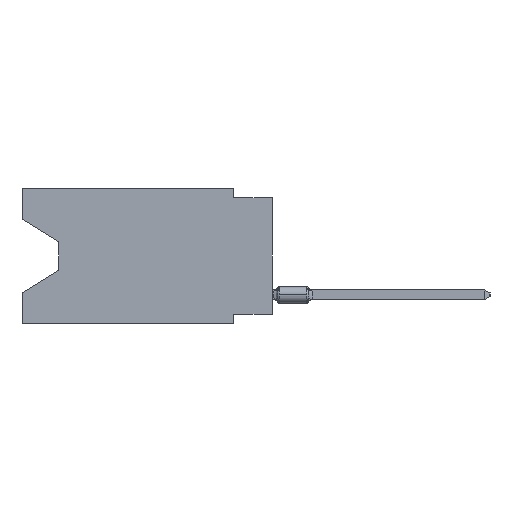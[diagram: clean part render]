
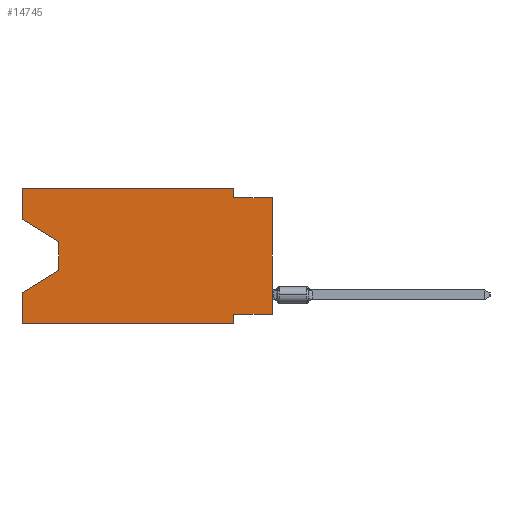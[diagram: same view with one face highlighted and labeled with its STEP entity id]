
A CAD part, left-side view. The second image highlights one B-rep face of the part: STEP entity #14745.
In plain terms, the highlighted planar face has unit normal (-1, 0, 0).
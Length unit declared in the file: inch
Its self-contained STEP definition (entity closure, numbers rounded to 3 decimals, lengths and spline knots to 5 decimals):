
#199 = ORIENTED_EDGE ( 'NONE', *, *, #22991, .T. ) ;
#1164 = CARTESIAN_POINT ( 'NONE',  ( 0., 0., -0.025 ) ) ;
#1546 = VERTEX_POINT ( 'NONE', #31990 ) ;
#1868 = CARTESIAN_POINT ( 'NONE',  ( 0., 0.645, 0. ) ) ;
#2002 = LINE ( 'NONE', #14101, #34055 ) ;
#2009 = VECTOR ( 'NONE', #32151, 39.37008 ) ;
#3242 = EDGE_CURVE ( 'NONE', #35832, #35520, #16876, .T. ) ;
#3734 = EDGE_CURVE ( 'NONE', #18222, #15809, #5132, .T. ) ;
#4199 = VERTEX_POINT ( 'NONE', #38492 ) ;
#4399 = CARTESIAN_POINT ( 'NONE',  ( 0., 0.1, -0.325 ) ) ;
#4623 = CARTESIAN_POINT ( 'NONE',  ( 0., 0., -0.325 ) ) ;
#4688 = EDGE_CURVE ( 'NONE', #5447, #1546, #36260, .T. ) ;
#5040 = CARTESIAN_POINT ( 'NONE',  ( 0., 0.645, -0.08025 ) ) ;
#5132 = LINE ( 'NONE', #23923, #17165 ) ;
#5334 = ORIENTED_EDGE ( 'NONE', *, *, #19555, .T. ) ;
#5447 = VERTEX_POINT ( 'NONE', #22988 ) ;
#5611 = DIRECTION ( 'NONE',  ( 0., -1., 0. ) ) ;
#5726 = VERTEX_POINT ( 'NONE', #40575 ) ;
#6654 = LINE ( 'NONE', #32352, #2009 ) ;
#6931 = LINE ( 'NONE', #4623, #17175 ) ;
#7635 = DIRECTION ( 'NONE',  ( 0., -1., 0. ) ) ;
#8269 = DIRECTION ( 'NONE',  ( 0., 0., -1. ) ) ;
#8431 = DIRECTION ( 'NONE',  ( 0., 0., -1. ) ) ;
#8499 = VERTEX_POINT ( 'NONE', #1868 ) ;
#9174 = ORIENTED_EDGE ( 'NONE', *, *, #12309, .T. ) ;
#11509 = ORIENTED_EDGE ( 'NONE', *, *, #4688, .F. ) ;
#12097 = EDGE_CURVE ( 'NONE', #13917, #1546, #31571, .T. ) ;
#12309 = EDGE_CURVE ( 'NONE', #35520, #5726, #17955, .T. ) ;
#12807 = VERTEX_POINT ( 'NONE', #15783 ) ;
#13898 = VECTOR ( 'NONE', #21727, 39.37008 ) ;
#13917 = VERTEX_POINT ( 'NONE', #22105 ) ;
#14101 = CARTESIAN_POINT ( 'NONE',  ( 0., 0.1, 0. ) ) ;
#14236 = LINE ( 'NONE', #5040, #26431 ) ;
#14745 = ADVANCED_FACE ( 'NONE', ( #33713 ), #17830, .F. ) ;
#14807 = ORIENTED_EDGE ( 'NONE', *, *, #16747, .F. ) ;
#15742 = AXIS2_PLACEMENT_3D ( 'NONE', #30992, #30579, #8431 ) ;
#15783 = CARTESIAN_POINT ( 'NONE',  ( 0., 0.1, 0. ) ) ;
#15809 = VERTEX_POINT ( 'NONE', #36436 ) ;
#16140 = EDGE_LOOP ( 'NONE', ( #5334, #34953, #9174, #19486, #199, #28692, #25940, #30417, #11509, #25548, #23021, #14807 ) ) ;
#16747 = EDGE_CURVE ( 'NONE', #23417, #8499, #40895, .T. ) ;
#16876 = LINE ( 'NONE', #17291, #36505 ) ;
#17165 = VECTOR ( 'NONE', #8269, 39.37008 ) ;
#17175 = VECTOR ( 'NONE', #38710, 39.37008 ) ;
#17291 = CARTESIAN_POINT ( 'NONE',  ( 0., 0.55, -0.138 ) ) ;
#17830 = PLANE ( 'NONE',  #15742 ) ;
#17949 = VECTOR ( 'NONE', #31971, 39.37008 ) ;
#17955 = LINE ( 'NONE', #40117, #21286 ) ;
#18222 = VERTEX_POINT ( 'NONE', #4399 ) ;
#19486 = ORIENTED_EDGE ( 'NONE', *, *, #25926, .F. ) ;
#19555 = EDGE_CURVE ( 'NONE', #23417, #35832, #14236, .T. ) ;
#21214 = DIRECTION ( 'NONE',  ( 0., 0., -1. ) ) ;
#21286 = VECTOR ( 'NONE', #39903, 39.37008 ) ;
#21301 = EDGE_CURVE ( 'NONE', #13917, #18222, #6931, .T. ) ;
#21727 = DIRECTION ( 'NONE',  ( 0., -1., 0. ) ) ;
#21840 = CARTESIAN_POINT ( 'NONE',  ( 0., 0.645, 0. ) ) ;
#22105 = CARTESIAN_POINT ( 'NONE',  ( 0., 0., -0.325 ) ) ;
#22341 = CARTESIAN_POINT ( 'NONE',  ( 0., 0., 0. ) ) ;
#22583 = EDGE_CURVE ( 'NONE', #8499, #12807, #34102, .T. ) ;
#22988 = CARTESIAN_POINT ( 'NONE',  ( 0., 0.1, -0.025 ) ) ;
#22991 = EDGE_CURVE ( 'NONE', #4199, #15809, #28363, .T. ) ;
#23021 = ORIENTED_EDGE ( 'NONE', *, *, #22583, .F. ) ;
#23417 = VERTEX_POINT ( 'NONE', #30860 ) ;
#23923 = CARTESIAN_POINT ( 'NONE',  ( 0., 0.1, -0.35 ) ) ;
#25548 = ORIENTED_EDGE ( 'NONE', *, *, #26018, .F. ) ;
#25926 = EDGE_CURVE ( 'NONE', #4199, #5726, #6654, .T. ) ;
#25940 = ORIENTED_EDGE ( 'NONE', *, *, #21301, .F. ) ;
#26018 = EDGE_CURVE ( 'NONE', #12807, #5447, #2002, .T. ) ;
#26266 = DIRECTION ( 'NONE',  ( 0., 0., -1. ) ) ;
#26302 = CARTESIAN_POINT ( 'NONE',  ( 0., 0.55, -0.212 ) ) ;
#26431 = VECTOR ( 'NONE', #40162, 39.37008 ) ;
#28021 = CARTESIAN_POINT ( 'NONE',  ( 0., 0.645, 0. ) ) ;
#28363 = LINE ( 'NONE', #41143, #37423 ) ;
#28692 = ORIENTED_EDGE ( 'NONE', *, *, #3734, .F. ) ;
#29399 = CARTESIAN_POINT ( 'NONE',  ( 0., 0.55, -0.138 ) ) ;
#30417 = ORIENTED_EDGE ( 'NONE', *, *, #12097, .T. ) ;
#30579 = DIRECTION ( 'NONE',  ( 1., 0., 0. ) ) ;
#30860 = CARTESIAN_POINT ( 'NONE',  ( 0., 0.645, -0.08025 ) ) ;
#30992 = CARTESIAN_POINT ( 'NONE',  ( 0., 0.645, 0. ) ) ;
#31571 = LINE ( 'NONE', #22341, #17949 ) ;
#31971 = DIRECTION ( 'NONE',  ( 0., 0., 1. ) ) ;
#31990 = CARTESIAN_POINT ( 'NONE',  ( 0., 0., -0.025 ) ) ;
#32151 = DIRECTION ( 'NONE',  ( 0., 0., 1. ) ) ;
#32352 = CARTESIAN_POINT ( 'NONE',  ( 0., 0.645, 0. ) ) ;
#32819 = VECTOR ( 'NONE', #7635, 39.37008 ) ;
#33041 = VECTOR ( 'NONE', #34401, 39.37008 ) ;
#33713 = FACE_OUTER_BOUND ( 'NONE', #16140, .T. ) ;
#34055 = VECTOR ( 'NONE', #21214, 39.37008 ) ;
#34102 = LINE ( 'NONE', #28021, #13898 ) ;
#34401 = DIRECTION ( 'NONE',  ( 0., 0., 1. ) ) ;
#34953 = ORIENTED_EDGE ( 'NONE', *, *, #3242, .T. ) ;
#35520 = VERTEX_POINT ( 'NONE', #26302 ) ;
#35832 = VERTEX_POINT ( 'NONE', #29399 ) ;
#36260 = LINE ( 'NONE', #1164, #32819 ) ;
#36436 = CARTESIAN_POINT ( 'NONE',  ( 0., 0.1, -0.35 ) ) ;
#36505 = VECTOR ( 'NONE', #26266, 39.37008 ) ;
#37423 = VECTOR ( 'NONE', #5611, 39.37008 ) ;
#38492 = CARTESIAN_POINT ( 'NONE',  ( 0., 0.645, -0.35 ) ) ;
#38710 = DIRECTION ( 'NONE',  ( 0., 1., 0. ) ) ;
#39903 = DIRECTION ( 'NONE',  ( 0., 0.855, -0.519 ) ) ;
#40117 = CARTESIAN_POINT ( 'NONE',  ( 0., 0.55, -0.212 ) ) ;
#40162 = DIRECTION ( 'NONE',  ( 0., -0.855, -0.519 ) ) ;
#40575 = CARTESIAN_POINT ( 'NONE',  ( 0., 0.645, -0.26975 ) ) ;
#40895 = LINE ( 'NONE', #21840, #33041 ) ;
#41143 = CARTESIAN_POINT ( 'NONE',  ( 0., 0.645, -0.35 ) ) ;
